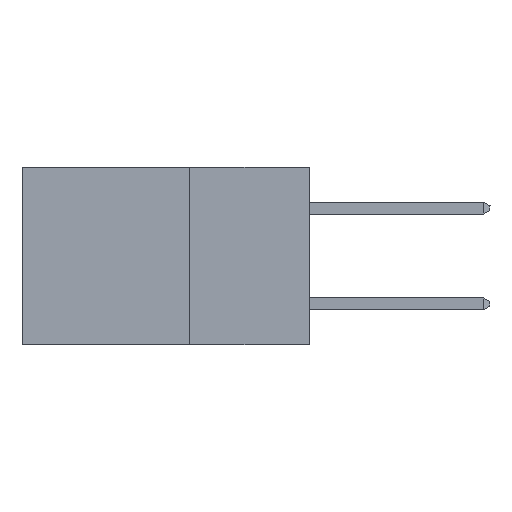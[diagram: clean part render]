
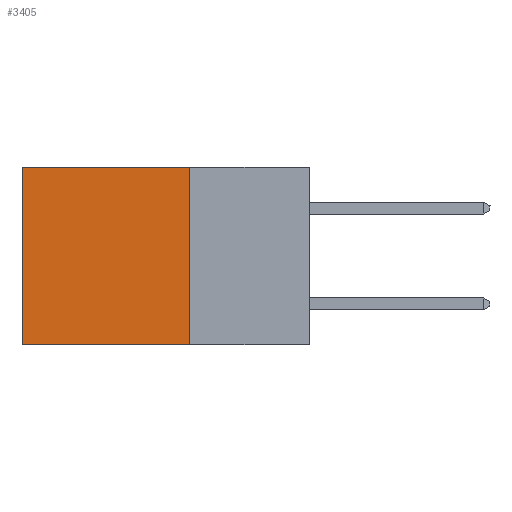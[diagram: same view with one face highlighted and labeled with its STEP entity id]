
A CAD part, left-side view. The second image highlights one B-rep face of the part: STEP entity #3405.
In plain terms, the highlighted planar face has unit normal (-1, 0, 0).
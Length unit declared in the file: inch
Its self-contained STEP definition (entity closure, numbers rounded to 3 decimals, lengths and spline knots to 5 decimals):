
#86 = EDGE_CURVE ( 'NONE', #8831, #2154, #4518, .T. ) ;
#232 = CARTESIAN_POINT ( 'NONE',  ( 0.2875, 0.6, -0.37 ) ) ;
#417 = CARTESIAN_POINT ( 'NONE',  ( 0.2875, 0.6, 0. ) ) ;
#700 = LINE ( 'NONE', #2575, #7810 ) ;
#707 = CARTESIAN_POINT ( 'NONE',  ( 0.2875, 0.25, -0.37 ) ) ;
#952 = DIRECTION ( 'NONE',  ( 0., 1., 0. ) ) ;
#1255 = DIRECTION ( 'NONE',  ( 0., 1., 0. ) ) ;
#2154 = VERTEX_POINT ( 'NONE', #9467 ) ;
#2575 = CARTESIAN_POINT ( 'NONE',  ( 0.2875, 0.25, -0.37 ) ) ;
#2911 = PLANE ( 'NONE',  #7952 ) ;
#3097 = ORIENTED_EDGE ( 'NONE', *, *, #10066, .F. ) ;
#3405 = ADVANCED_FACE ( 'NONE', ( #10715 ), #2911, .F. ) ;
#3513 = CARTESIAN_POINT ( 'NONE',  ( 0.2875, 0.25, 0. ) ) ;
#4518 = LINE ( 'NONE', #4802, #6294 ) ;
#4622 = LINE ( 'NONE', #3513, #5732 ) ;
#4802 = CARTESIAN_POINT ( 'NONE',  ( 0.2875, 0.25, 0. ) ) ;
#5190 = LINE ( 'NONE', #417, #6285 ) ;
#5387 = DIRECTION ( 'NONE',  ( 0., 0., -1. ) ) ;
#5732 = VECTOR ( 'NONE', #6070, 39.37008 ) ;
#6070 = DIRECTION ( 'NONE',  ( 0., 0., -1. ) ) ;
#6285 = VECTOR ( 'NONE', #9585, 39.37008 ) ;
#6294 = VECTOR ( 'NONE', #1255, 39.37008 ) ;
#6351 = CARTESIAN_POINT ( 'NONE',  ( 0.2875, 0.25, 0. ) ) ;
#6358 = VERTEX_POINT ( 'NONE', #707 ) ;
#7650 = ORIENTED_EDGE ( 'NONE', *, *, #10276, .F. ) ;
#7810 = VECTOR ( 'NONE', #952, 39.37008 ) ;
#7952 = AXIS2_PLACEMENT_3D ( 'NONE', #9710, #8039, #5387 ) ;
#7987 = VERTEX_POINT ( 'NONE', #232 ) ;
#8039 = DIRECTION ( 'NONE',  ( 1., 0., 0. ) ) ;
#8103 = EDGE_CURVE ( 'NONE', #2154, #7987, #5190, .T. ) ;
#8831 = VERTEX_POINT ( 'NONE', #6351 ) ;
#9467 = CARTESIAN_POINT ( 'NONE',  ( 0.2875, 0.6, 0. ) ) ;
#9585 = DIRECTION ( 'NONE',  ( 0., 0., -1. ) ) ;
#9710 = CARTESIAN_POINT ( 'NONE',  ( 0.2875, 0.25, 0. ) ) ;
#10066 = EDGE_CURVE ( 'NONE', #8831, #6358, #4622, .T. ) ;
#10105 = ORIENTED_EDGE ( 'NONE', *, *, #86, .T. ) ;
#10276 = EDGE_CURVE ( 'NONE', #6358, #7987, #700, .T. ) ;
#10474 = EDGE_LOOP ( 'NONE', ( #10861, #7650, #3097, #10105 ) ) ;
#10715 = FACE_OUTER_BOUND ( 'NONE', #10474, .T. ) ;
#10861 = ORIENTED_EDGE ( 'NONE', *, *, #8103, .T. ) ;
